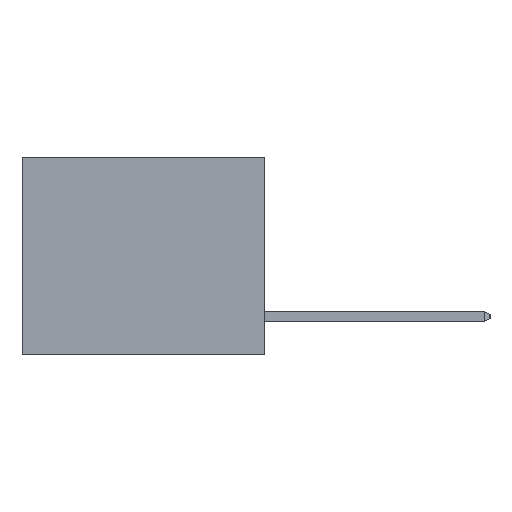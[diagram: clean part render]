
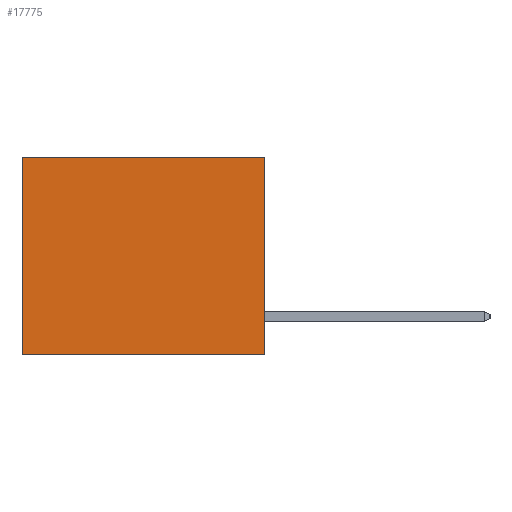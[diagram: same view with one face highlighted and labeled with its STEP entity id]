
A CAD part, left-side view. The second image highlights one B-rep face of the part: STEP entity #17775.
In plain terms, the highlighted planar face has unit normal (-1, 0, 0).
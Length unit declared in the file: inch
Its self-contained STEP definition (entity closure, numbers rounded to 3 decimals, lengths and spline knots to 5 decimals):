
#417 = DIRECTION ( 'NONE',  ( 0., 1., 0. ) ) ;
#698 = DIRECTION ( 'NONE',  ( 0., 0., -1. ) ) ;
#1605 = DIRECTION ( 'NONE',  ( 0., 0., -1. ) ) ;
#1881 = CARTESIAN_POINT ( 'NONE',  ( 0.3165, 0.6, 0. ) ) ;
#1904 = ORIENTED_EDGE ( 'NONE', *, *, #3664, .T. ) ;
#2347 = VERTEX_POINT ( 'NONE', #19474 ) ;
#3449 = DIRECTION ( 'NONE',  ( 0., 1., 0. ) ) ;
#3664 = EDGE_CURVE ( 'NONE', #13369, #14422, #4509, .T. ) ;
#4509 = LINE ( 'NONE', #19320, #8802 ) ;
#6422 = CARTESIAN_POINT ( 'NONE',  ( 0.3165, 0., 0. ) ) ;
#6759 = VECTOR ( 'NONE', #8856, 39.37008 ) ;
#7367 = PLANE ( 'NONE',  #19478 ) ;
#7442 = CARTESIAN_POINT ( 'NONE',  ( 0.3165, 0., -0.49 ) ) ;
#8369 = CARTESIAN_POINT ( 'NONE',  ( 0.3165, 0., -0.49 ) ) ;
#8792 = CARTESIAN_POINT ( 'NONE',  ( 0.3165, 0., -0.49 ) ) ;
#8802 = VECTOR ( 'NONE', #1605, 39.37008 ) ;
#8856 = DIRECTION ( 'NONE',  ( 0., 0., -1. ) ) ;
#9104 = DIRECTION ( 'NONE',  ( 1., 0., 0. ) ) ;
#10321 = FACE_OUTER_BOUND ( 'NONE', #17649, .T. ) ;
#10412 = LINE ( 'NONE', #14977, #19076 ) ;
#10564 = CARTESIAN_POINT ( 'NONE',  ( 0.3165, 0.6, -0.49 ) ) ;
#10632 = LINE ( 'NONE', #8792, #6759 ) ;
#10906 = EDGE_CURVE ( 'NONE', #19222, #14422, #10412, .T. ) ;
#11588 = ORIENTED_EDGE ( 'NONE', *, *, #12013, .F. ) ;
#12013 = EDGE_CURVE ( 'NONE', #2347, #19222, #10632, .T. ) ;
#13369 = VERTEX_POINT ( 'NONE', #1881 ) ;
#14422 = VERTEX_POINT ( 'NONE', #10564 ) ;
#14977 = CARTESIAN_POINT ( 'NONE',  ( 0.3165, 0., -0.49 ) ) ;
#16139 = LINE ( 'NONE', #6422, #17943 ) ;
#17649 = EDGE_LOOP ( 'NONE', ( #1904, #20252, #11588, #18104 ) ) ;
#17775 = ADVANCED_FACE ( 'NONE', ( #10321 ), #7367, .F. ) ;
#17943 = VECTOR ( 'NONE', #3449, 39.37008 ) ;
#18104 = ORIENTED_EDGE ( 'NONE', *, *, #18248, .T. ) ;
#18248 = EDGE_CURVE ( 'NONE', #2347, #13369, #16139, .T. ) ;
#19076 = VECTOR ( 'NONE', #417, 39.37008 ) ;
#19222 = VERTEX_POINT ( 'NONE', #8369 ) ;
#19320 = CARTESIAN_POINT ( 'NONE',  ( 0.3165, 0.6, -0.49 ) ) ;
#19474 = CARTESIAN_POINT ( 'NONE',  ( 0.3165, 0., 0. ) ) ;
#19478 = AXIS2_PLACEMENT_3D ( 'NONE', #7442, #9104, #698 ) ;
#20252 = ORIENTED_EDGE ( 'NONE', *, *, #10906, .F. ) ;
